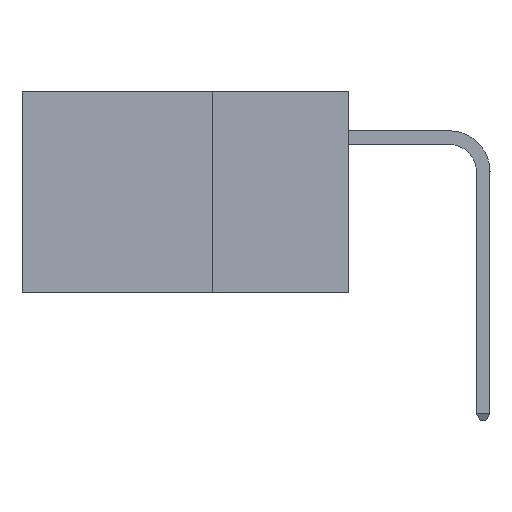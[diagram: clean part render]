
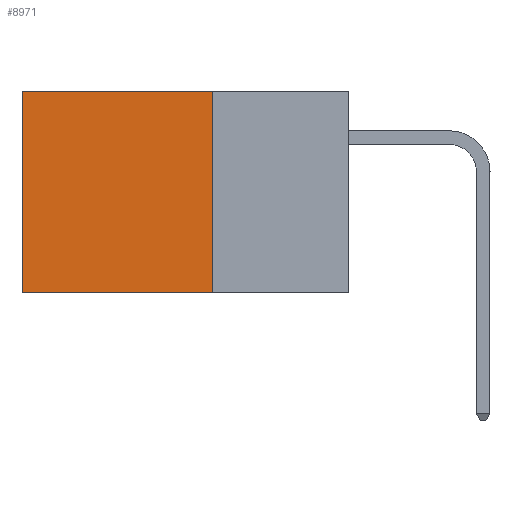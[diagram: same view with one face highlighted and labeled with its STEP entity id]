
A CAD part, left-side view. The second image highlights one B-rep face of the part: STEP entity #8971.
In plain terms, the highlighted planar face has unit normal (-1, 0, 0).
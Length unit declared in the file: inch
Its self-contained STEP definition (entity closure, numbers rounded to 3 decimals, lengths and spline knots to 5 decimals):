
#460 = CARTESIAN_POINT ( 'NONE',  ( 0.2875, 0.6, 0. ) ) ;
#1577 = DIRECTION ( 'NONE',  ( 0., 1., 0. ) ) ;
#2317 = PLANE ( 'NONE',  #37740 ) ;
#2672 = VECTOR ( 'NONE', #1577, 39.37008 ) ;
#3754 = VECTOR ( 'NONE', #25194, 39.37008 ) ;
#4179 = CARTESIAN_POINT ( 'NONE',  ( 0.2875, 0.6, 0. ) ) ;
#4842 = CARTESIAN_POINT ( 'NONE',  ( 0.2875, 0.6, -0.37 ) ) ;
#5881 = CARTESIAN_POINT ( 'NONE',  ( 0.2875, 0.25, 0. ) ) ;
#8642 = EDGE_CURVE ( 'NONE', #35682, #40208, #33759, .T. ) ;
#8792 = ORIENTED_EDGE ( 'NONE', *, *, #18660, .F. ) ;
#8971 = ADVANCED_FACE ( 'NONE', ( #30941 ), #2317, .F. ) ;
#9448 = DIRECTION ( 'NONE',  ( 1., 0., 0. ) ) ;
#14458 = EDGE_LOOP ( 'NONE', ( #24834, #42555, #8792, #28097 ) ) ;
#14713 = DIRECTION ( 'NONE',  ( 0., 0., -1. ) ) ;
#18660 = EDGE_CURVE ( 'NONE', #35682, #31336, #33131, .T. ) ;
#20459 = CARTESIAN_POINT ( 'NONE',  ( 0.2875, 0.25, 0. ) ) ;
#21639 = CARTESIAN_POINT ( 'NONE',  ( 0.2875, 0.25, 0. ) ) ;
#21832 = CARTESIAN_POINT ( 'NONE',  ( 0.2875, 0.25, 0. ) ) ;
#24834 = ORIENTED_EDGE ( 'NONE', *, *, #40158, .T. ) ;
#25194 = DIRECTION ( 'NONE',  ( 0., 0., -1. ) ) ;
#25344 = LINE ( 'NONE', #460, #32541 ) ;
#25419 = DIRECTION ( 'NONE',  ( 0., 1., 0. ) ) ;
#28097 = ORIENTED_EDGE ( 'NONE', *, *, #8642, .T. ) ;
#28914 = EDGE_CURVE ( 'NONE', #31336, #35412, #40353, .T. ) ;
#30941 = FACE_OUTER_BOUND ( 'NONE', #14458, .T. ) ;
#31336 = VERTEX_POINT ( 'NONE', #41367 ) ;
#32541 = VECTOR ( 'NONE', #14713, 39.37008 ) ;
#32628 = VECTOR ( 'NONE', #25419, 39.37008 ) ;
#33131 = LINE ( 'NONE', #21639, #3754 ) ;
#33327 = CARTESIAN_POINT ( 'NONE',  ( 0.2875, 0.25, -0.37 ) ) ;
#33759 = LINE ( 'NONE', #21832, #32628 ) ;
#34225 = DIRECTION ( 'NONE',  ( 0., 0., -1. ) ) ;
#35412 = VERTEX_POINT ( 'NONE', #4842 ) ;
#35682 = VERTEX_POINT ( 'NONE', #20459 ) ;
#37740 = AXIS2_PLACEMENT_3D ( 'NONE', #5881, #9448, #34225 ) ;
#40158 = EDGE_CURVE ( 'NONE', #40208, #35412, #25344, .T. ) ;
#40208 = VERTEX_POINT ( 'NONE', #4179 ) ;
#40353 = LINE ( 'NONE', #33327, #2672 ) ;
#41367 = CARTESIAN_POINT ( 'NONE',  ( 0.2875, 0.25, -0.37 ) ) ;
#42555 = ORIENTED_EDGE ( 'NONE', *, *, #28914, .F. ) ;
